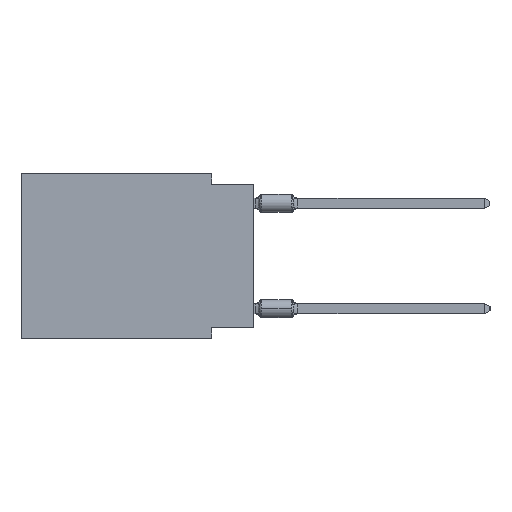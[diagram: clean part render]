
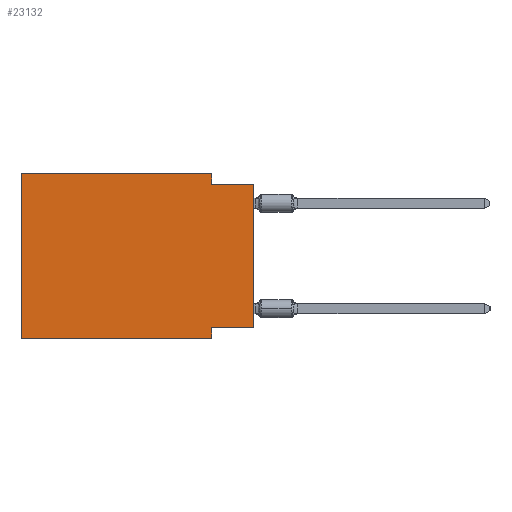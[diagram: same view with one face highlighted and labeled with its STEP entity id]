
A CAD part, left-side view. The second image highlights one B-rep face of the part: STEP entity #23132.
In plain terms, the highlighted planar face has unit normal (-1, 0, 0).
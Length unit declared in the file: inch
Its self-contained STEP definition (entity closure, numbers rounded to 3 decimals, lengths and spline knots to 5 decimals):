
#1140 = CARTESIAN_POINT ( 'NONE',  ( 0., 0.55, -0.39 ) ) ;
#1266 = VECTOR ( 'NONE', #31789, 39.37008 ) ;
#1472 = DIRECTION ( 'NONE',  ( 0., 1., 0. ) ) ;
#2126 = EDGE_CURVE ( 'NONE', #20944, #39727, #29337, .T. ) ;
#2764 = CARTESIAN_POINT ( 'NONE',  ( 0., 0.55, 0. ) ) ;
#6918 = EDGE_LOOP ( 'NONE', ( #11733, #19870, #17956, #16834, #11261, #42377, #23019, #20143 ) ) ;
#8668 = CARTESIAN_POINT ( 'NONE',  ( 0., 0.1, 0. ) ) ;
#10055 = VECTOR ( 'NONE', #35963, 39.37008 ) ;
#11261 = ORIENTED_EDGE ( 'NONE', *, *, #35897, .F. ) ;
#11733 = ORIENTED_EDGE ( 'NONE', *, *, #20921, .T. ) ;
#11904 = EDGE_CURVE ( 'NONE', #39727, #34406, #35654, .T. ) ;
#12466 = CARTESIAN_POINT ( 'NONE',  ( 0., 0.55, -0.39 ) ) ;
#12699 = CARTESIAN_POINT ( 'NONE',  ( 0., 0.55, 0. ) ) ;
#12903 = DIRECTION ( 'NONE',  ( 0., -1., 0. ) ) ;
#12942 = FACE_OUTER_BOUND ( 'NONE', #6918, .T. ) ;
#13590 = VERTEX_POINT ( 'NONE', #43087 ) ;
#13995 = CARTESIAN_POINT ( 'NONE',  ( 0., 0.1, 0. ) ) ;
#15147 = EDGE_CURVE ( 'NONE', #32868, #19887, #15183, .T. ) ;
#15183 = LINE ( 'NONE', #28503, #25930 ) ;
#15968 = VECTOR ( 'NONE', #12903, 39.37008 ) ;
#16283 = DIRECTION ( 'NONE',  ( 1., 0., 0. ) ) ;
#16665 = EDGE_CURVE ( 'NONE', #34406, #13590, #38191, .T. ) ;
#16834 = ORIENTED_EDGE ( 'NONE', *, *, #2126, .F. ) ;
#17956 = ORIENTED_EDGE ( 'NONE', *, *, #11904, .F. ) ;
#18389 = VECTOR ( 'NONE', #39472, 39.37008 ) ;
#19799 = DIRECTION ( 'NONE',  ( 0., 0., 1. ) ) ;
#19870 = ORIENTED_EDGE ( 'NONE', *, *, #16665, .F. ) ;
#19887 = VERTEX_POINT ( 'NONE', #21354 ) ;
#20143 = ORIENTED_EDGE ( 'NONE', *, *, #15147, .F. ) ;
#20156 = EDGE_CURVE ( 'NONE', #19887, #39977, #29724, .T. ) ;
#20241 = CARTESIAN_POINT ( 'NONE',  ( 0., 0.55, 0. ) ) ;
#20921 = EDGE_CURVE ( 'NONE', #32868, #13590, #29783, .T. ) ;
#20944 = VERTEX_POINT ( 'NONE', #20241 ) ;
#21354 = CARTESIAN_POINT ( 'NONE',  ( 0., 0.1, -0.365 ) ) ;
#21378 = AXIS2_PLACEMENT_3D ( 'NONE', #2764, #16283, #22297 ) ;
#21499 = CARTESIAN_POINT ( 'NONE',  ( 0., 0.1, -0.39 ) ) ;
#22083 = PLANE ( 'NONE',  #21378 ) ;
#22114 = VECTOR ( 'NONE', #24200, 39.37008 ) ;
#22297 = DIRECTION ( 'NONE',  ( 0., 0., -1. ) ) ;
#23019 = ORIENTED_EDGE ( 'NONE', *, *, #20156, .F. ) ;
#23132 = ADVANCED_FACE ( 'NONE', ( #12942 ), #22083, .F. ) ;
#23439 = EDGE_CURVE ( 'NONE', #37124, #39977, #32433, .T. ) ;
#24200 = DIRECTION ( 'NONE',  ( 0., 0., -1. ) ) ;
#25930 = VECTOR ( 'NONE', #1472, 39.37008 ) ;
#26862 = CARTESIAN_POINT ( 'NONE',  ( 0., 0., -0.365 ) ) ;
#27300 = CARTESIAN_POINT ( 'NONE',  ( 0., 0.55, 0. ) ) ;
#28503 = CARTESIAN_POINT ( 'NONE',  ( 0., 0., -0.365 ) ) ;
#29337 = LINE ( 'NONE', #12699, #15968 ) ;
#29709 = VECTOR ( 'NONE', #19799, 39.37008 ) ;
#29724 = LINE ( 'NONE', #29933, #18389 ) ;
#29783 = LINE ( 'NONE', #29993, #29709 ) ;
#29933 = CARTESIAN_POINT ( 'NONE',  ( 0., 0.1, -0.39 ) ) ;
#29993 = CARTESIAN_POINT ( 'NONE',  ( 0., 0., 0. ) ) ;
#31782 = CARTESIAN_POINT ( 'NONE',  ( 0., 0.1, -0.025 ) ) ;
#31789 = DIRECTION ( 'NONE',  ( 0., -1., 0. ) ) ;
#32433 = LINE ( 'NONE', #12466, #10055 ) ;
#32868 = VERTEX_POINT ( 'NONE', #26862 ) ;
#34406 = VERTEX_POINT ( 'NONE', #31782 ) ;
#35532 = CARTESIAN_POINT ( 'NONE',  ( 0., 0., -0.025 ) ) ;
#35654 = LINE ( 'NONE', #13995, #22114 ) ;
#35897 = EDGE_CURVE ( 'NONE', #37124, #20944, #37471, .T. ) ;
#35963 = DIRECTION ( 'NONE',  ( 0., -1., 0. ) ) ;
#37124 = VERTEX_POINT ( 'NONE', #1140 ) ;
#37471 = LINE ( 'NONE', #27300, #40777 ) ;
#38191 = LINE ( 'NONE', #35532, #1266 ) ;
#39472 = DIRECTION ( 'NONE',  ( 0., 0., -1. ) ) ;
#39727 = VERTEX_POINT ( 'NONE', #8668 ) ;
#39977 = VERTEX_POINT ( 'NONE', #21499 ) ;
#40777 = VECTOR ( 'NONE', #40788, 39.37008 ) ;
#40788 = DIRECTION ( 'NONE',  ( 0., 0., 1. ) ) ;
#42377 = ORIENTED_EDGE ( 'NONE', *, *, #23439, .T. ) ;
#43087 = CARTESIAN_POINT ( 'NONE',  ( 0., 0., -0.025 ) ) ;
